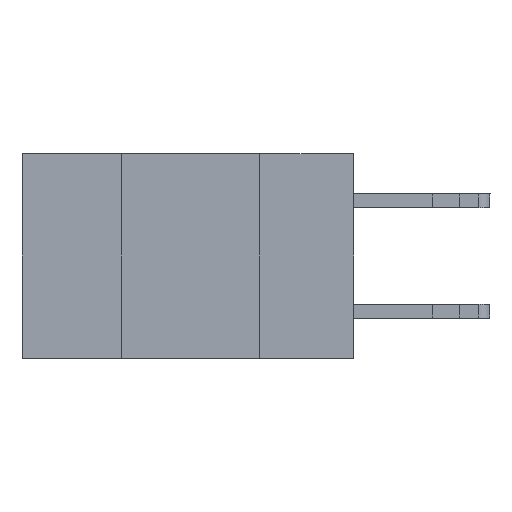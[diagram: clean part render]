
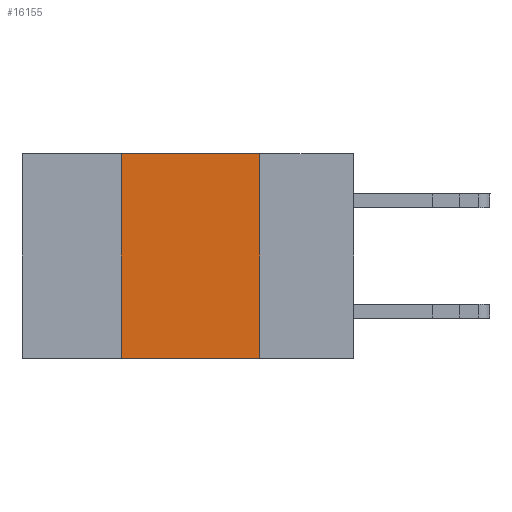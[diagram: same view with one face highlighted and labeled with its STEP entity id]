
A CAD part, left-side view. The second image highlights one B-rep face of the part: STEP entity #16155.
In plain terms, the highlighted planar face has unit normal (-1, 0, 0).
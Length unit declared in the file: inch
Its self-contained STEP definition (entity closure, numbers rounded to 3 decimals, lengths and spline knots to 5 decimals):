
#261 = DIRECTION ( 'NONE',  ( 0., 0., -1. ) ) ;
#660 = VERTEX_POINT ( 'NONE', #18550 ) ;
#2588 = CARTESIAN_POINT ( 'NONE',  ( 0., 0.6, 0. ) ) ;
#4171 = VERTEX_POINT ( 'NONE', #23291 ) ;
#5523 = VECTOR ( 'NONE', #27619, 39.37008 ) ;
#7580 = VERTEX_POINT ( 'NONE', #11044 ) ;
#7630 = FACE_OUTER_BOUND ( 'NONE', #8755, .T. ) ;
#8581 = VECTOR ( 'NONE', #26146, 39.37008 ) ;
#8755 = EDGE_LOOP ( 'NONE', ( #8848, #13382, #21371, #11699 ) ) ;
#8848 = ORIENTED_EDGE ( 'NONE', *, *, #15083, .F. ) ;
#11044 = CARTESIAN_POINT ( 'NONE',  ( 0., 0.42, -0.37 ) ) ;
#11386 = DIRECTION ( 'NONE',  ( 1., 0., 0. ) ) ;
#11699 = ORIENTED_EDGE ( 'NONE', *, *, #26313, .T. ) ;
#12077 = EDGE_CURVE ( 'NONE', #7580, #660, #21045, .T. ) ;
#12128 = CARTESIAN_POINT ( 'NONE',  ( 0., 0.17, 0. ) ) ;
#13382 = ORIENTED_EDGE ( 'NONE', *, *, #16967, .F. ) ;
#13914 = CARTESIAN_POINT ( 'NONE',  ( 0., 0.17, -0.37 ) ) ;
#13940 = DIRECTION ( 'NONE',  ( 0., -1., 0. ) ) ;
#15083 = EDGE_CURVE ( 'NONE', #4171, #17581, #17328, .T. ) ;
#15438 = LINE ( 'NONE', #2588, #27612 ) ;
#16155 = ADVANCED_FACE ( 'NONE', ( #7630 ), #29505, .F. ) ;
#16967 = EDGE_CURVE ( 'NONE', #660, #4171, #15438, .T. ) ;
#17328 = LINE ( 'NONE', #12128, #25884 ) ;
#17581 = VERTEX_POINT ( 'NONE', #13914 ) ;
#18311 = CARTESIAN_POINT ( 'NONE',  ( 0., 0.6, -0.37 ) ) ;
#18550 = CARTESIAN_POINT ( 'NONE',  ( 0., 0.42, 0. ) ) ;
#19203 = DIRECTION ( 'NONE',  ( 0., 0., -1. ) ) ;
#20126 = AXIS2_PLACEMENT_3D ( 'NONE', #22852, #11386, #261 ) ;
#21045 = LINE ( 'NONE', #21462, #8581 ) ;
#21371 = ORIENTED_EDGE ( 'NONE', *, *, #12077, .F. ) ;
#21462 = CARTESIAN_POINT ( 'NONE',  ( 0., 0.42, 0. ) ) ;
#22852 = CARTESIAN_POINT ( 'NONE',  ( 0., 0.6, 0. ) ) ;
#23291 = CARTESIAN_POINT ( 'NONE',  ( 0., 0.17, 0. ) ) ;
#25884 = VECTOR ( 'NONE', #19203, 39.37008 ) ;
#26146 = DIRECTION ( 'NONE',  ( 0., 0., 1. ) ) ;
#26313 = EDGE_CURVE ( 'NONE', #7580, #17581, #27702, .T. ) ;
#27612 = VECTOR ( 'NONE', #13940, 39.37008 ) ;
#27619 = DIRECTION ( 'NONE',  ( 0., -1., 0. ) ) ;
#27702 = LINE ( 'NONE', #18311, #5523 ) ;
#29505 = PLANE ( 'NONE',  #20126 ) ;
